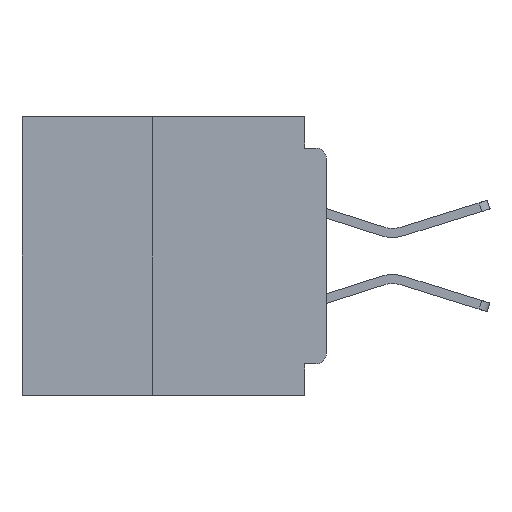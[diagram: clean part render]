
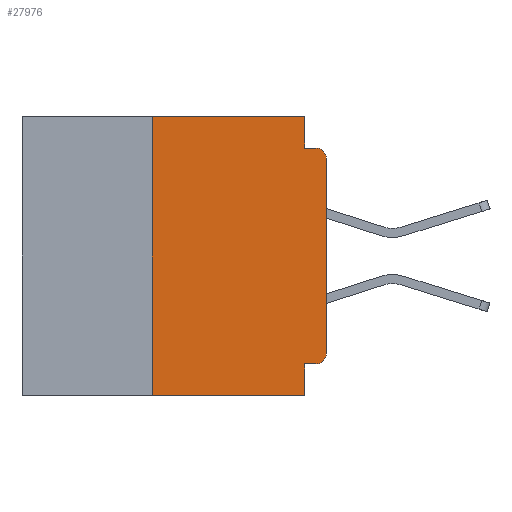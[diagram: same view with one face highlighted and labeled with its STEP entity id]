
A CAD part, left-side view. The second image highlights one B-rep face of the part: STEP entity #27976.
In plain terms, the highlighted planar face has unit normal (-1, 0, 0).
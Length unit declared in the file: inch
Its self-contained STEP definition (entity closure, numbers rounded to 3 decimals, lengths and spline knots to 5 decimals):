
#13 = EDGE_CURVE ( 'NONE', #38744, #27891, #36713, .T. ) ;
#701 = DIRECTION ( 'NONE',  ( 0., -1., 0. ) ) ;
#842 = ORIENTED_EDGE ( 'NONE', *, *, #36150, .T. ) ;
#1009 = CARTESIAN_POINT ( 'NONE',  ( 0., 0.031, -0.4 ) ) ;
#1387 = ORIENTED_EDGE ( 'NONE', *, *, #29127, .F. ) ;
#1806 = EDGE_CURVE ( 'NONE', #49971, #27891, #48195, .T. ) ;
#1962 = AXIS2_PLACEMENT_3D ( 'NONE', #49981, #26390, #2516 ) ;
#2516 = DIRECTION ( 'NONE',  ( 0., 0., -1. ) ) ;
#2710 = CARTESIAN_POINT ( 'NONE',  ( 0., 0., -0.045 ) ) ;
#3095 = LINE ( 'NONE', #38103, #33602 ) ;
#3217 = DIRECTION ( 'NONE',  ( 0., -1., 0. ) ) ;
#5421 = DIRECTION ( 'NONE',  ( 0., 0., -1. ) ) ;
#5759 = CARTESIAN_POINT ( 'NONE',  ( 0., 0.015, -0.355 ) ) ;
#6225 = ORIENTED_EDGE ( 'NONE', *, *, #14828, .F. ) ;
#6493 = CARTESIAN_POINT ( 'NONE',  ( 0., 0.031, -0.4 ) ) ;
#6520 = DIRECTION ( 'NONE',  ( 0., 1., 0. ) ) ;
#7088 = ORIENTED_EDGE ( 'NONE', *, *, #13, .T. ) ;
#7957 = VERTEX_POINT ( 'NONE', #6493 ) ;
#8156 = CARTESIAN_POINT ( 'NONE',  ( 0., 0.031, 0. ) ) ;
#8397 = VECTOR ( 'NONE', #3217, 39.37008 ) ;
#9154 = VECTOR ( 'NONE', #16845, 39.37008 ) ;
#9633 = ORIENTED_EDGE ( 'NONE', *, *, #13183, .T. ) ;
#9689 = LINE ( 'NONE', #15107, #8397 ) ;
#9866 = DIRECTION ( 'NONE',  ( 0., 0., -1. ) ) ;
#9907 = DIRECTION ( 'NONE',  ( -1., 0., 0. ) ) ;
#9917 = CARTESIAN_POINT ( 'NONE',  ( 0., 0.015, -0.06 ) ) ;
#10215 = ORIENTED_EDGE ( 'NONE', *, *, #29584, .T. ) ;
#12352 = CARTESIAN_POINT ( 'NONE',  ( 0., 0.437, 0. ) ) ;
#12446 = LINE ( 'NONE', #1009, #21738 ) ;
#12998 = CARTESIAN_POINT ( 'NONE',  ( 0., 0.015, -0.045 ) ) ;
#13183 = EDGE_CURVE ( 'NONE', #27625, #7957, #9689, .T. ) ;
#13234 = VECTOR ( 'NONE', #5421, 39.37008 ) ;
#13673 = DIRECTION ( 'NONE',  ( 0., 0., -1. ) ) ;
#13715 = FACE_OUTER_BOUND ( 'NONE', #30867, .T. ) ;
#14828 = EDGE_CURVE ( 'NONE', #19977, #49971, #44762, .T. ) ;
#15107 = CARTESIAN_POINT ( 'NONE',  ( 0., 0.437, -0.4 ) ) ;
#16845 = DIRECTION ( 'NONE',  ( 0., 0., 1. ) ) ;
#17805 = CARTESIAN_POINT ( 'NONE',  ( 0., 0.031, -0.355 ) ) ;
#19483 = EDGE_CURVE ( 'NONE', #34052, #7957, #12446, .T. ) ;
#19599 = CARTESIAN_POINT ( 'NONE',  ( 0., 0.25, -0.4 ) ) ;
#19977 = VERTEX_POINT ( 'NONE', #8156 ) ;
#20480 = DIRECTION ( 'NONE',  ( 0., -1., 0. ) ) ;
#20959 = LINE ( 'NONE', #48433, #9154 ) ;
#21325 = AXIS2_PLACEMENT_3D ( 'NONE', #9917, #9907, #9866 ) ;
#21449 = CARTESIAN_POINT ( 'NONE',  ( 0., 0.031, 0. ) ) ;
#21569 = CARTESIAN_POINT ( 'NONE',  ( 0., 0., 0. ) ) ;
#21616 = CARTESIAN_POINT ( 'NONE',  ( 0., 0.031, -0.045 ) ) ;
#21738 = VECTOR ( 'NONE', #28890, 39.37008 ) ;
#21920 = VECTOR ( 'NONE', #20480, 39.37008 ) ;
#23142 = CARTESIAN_POINT ( 'NONE',  ( 0., 0.25, 0. ) ) ;
#25467 = PLANE ( 'NONE',  #31224 ) ;
#26015 = EDGE_CURVE ( 'NONE', #26972, #19977, #32459, .T. ) ;
#26390 = DIRECTION ( 'NONE',  ( -1., 0., 0. ) ) ;
#26972 = VERTEX_POINT ( 'NONE', #23142 ) ;
#27272 = VECTOR ( 'NONE', #701, 39.37008 ) ;
#27625 = VERTEX_POINT ( 'NONE', #19599 ) ;
#27891 = VERTEX_POINT ( 'NONE', #12998 ) ;
#27976 = ADVANCED_FACE ( 'NONE', ( #13715 ), #25467, .F. ) ;
#28890 = DIRECTION ( 'NONE',  ( 0., 0., -1. ) ) ;
#28978 = ORIENTED_EDGE ( 'NONE', *, *, #26015, .F. ) ;
#29127 = EDGE_CURVE ( 'NONE', #27625, #26972, #20959, .T. ) ;
#29357 = VECTOR ( 'NONE', #41242, 39.37008 ) ;
#29584 = EDGE_CURVE ( 'NONE', #49959, #42522, #41908, .T. ) ;
#30867 = EDGE_LOOP ( 'NONE', ( #842, #7088, #30925, #6225, #28978, #1387, #9633, #34792, #40254, #10215 ) ) ;
#30925 = ORIENTED_EDGE ( 'NONE', *, *, #1806, .F. ) ;
#31224 = AXIS2_PLACEMENT_3D ( 'NONE', #49063, #37379, #13673 ) ;
#32459 = LINE ( 'NONE', #12352, #21920 ) ;
#33602 = VECTOR ( 'NONE', #6520, 39.37008 ) ;
#34052 = VERTEX_POINT ( 'NONE', #17805 ) ;
#34549 = CARTESIAN_POINT ( 'NONE',  ( 0., 0., -0.34 ) ) ;
#34792 = ORIENTED_EDGE ( 'NONE', *, *, #19483, .F. ) ;
#36150 = EDGE_CURVE ( 'NONE', #42522, #38744, #50275, .T. ) ;
#36713 = CIRCLE ( 'NONE', #21325, 0.015 ) ;
#37379 = DIRECTION ( 'NONE',  ( 1., 0., 0. ) ) ;
#38103 = CARTESIAN_POINT ( 'NONE',  ( 0., 0., -0.355 ) ) ;
#38744 = VERTEX_POINT ( 'NONE', #40291 ) ;
#40254 = ORIENTED_EDGE ( 'NONE', *, *, #45723, .F. ) ;
#40291 = CARTESIAN_POINT ( 'NONE',  ( 0., 0., -0.06 ) ) ;
#41242 = DIRECTION ( 'NONE',  ( 0., 0., 1. ) ) ;
#41908 = CIRCLE ( 'NONE', #1962, 0.015 ) ;
#42522 = VERTEX_POINT ( 'NONE', #34549 ) ;
#44762 = LINE ( 'NONE', #21449, #13234 ) ;
#45723 = EDGE_CURVE ( 'NONE', #49959, #34052, #3095, .T. ) ;
#48195 = LINE ( 'NONE', #2710, #27272 ) ;
#48433 = CARTESIAN_POINT ( 'NONE',  ( 0., 0.25, -0.4 ) ) ;
#49063 = CARTESIAN_POINT ( 'NONE',  ( 0., 0.437, 0. ) ) ;
#49959 = VERTEX_POINT ( 'NONE', #5759 ) ;
#49971 = VERTEX_POINT ( 'NONE', #21616 ) ;
#49981 = CARTESIAN_POINT ( 'NONE',  ( 0., 0.015, -0.34 ) ) ;
#50275 = LINE ( 'NONE', #21569, #29357 ) ;
